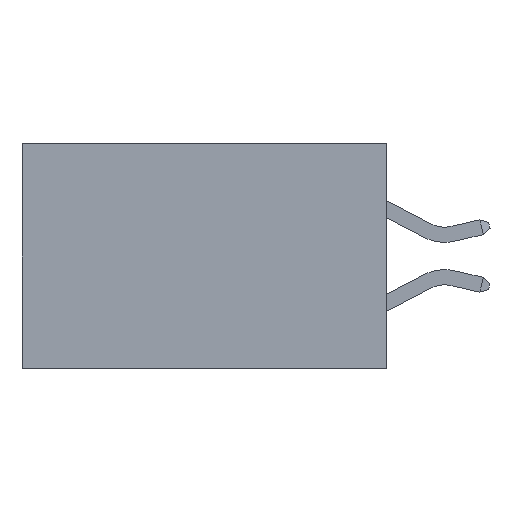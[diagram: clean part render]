
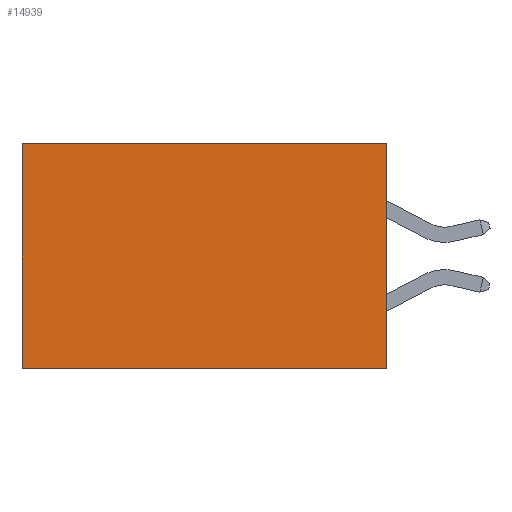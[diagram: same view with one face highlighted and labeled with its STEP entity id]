
A CAD part, left-side view. The second image highlights one B-rep face of the part: STEP entity #14939.
In plain terms, the highlighted planar face has unit normal (-1, 0, 0).
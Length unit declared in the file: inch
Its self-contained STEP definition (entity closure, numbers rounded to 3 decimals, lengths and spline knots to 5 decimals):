
#363 = DIRECTION ( 'NONE',  ( 0., 0., -1. ) ) ;
#607 = PLANE ( 'NONE',  #3276 ) ;
#1369 = DIRECTION ( 'NONE',  ( 0., 0., -1. ) ) ;
#1417 = VECTOR ( 'NONE', #17277, 39.37008 ) ;
#1928 = ORIENTED_EDGE ( 'NONE', *, *, #10941, .F. ) ;
#2033 = VERTEX_POINT ( 'NONE', #20275 ) ;
#2263 = ORIENTED_EDGE ( 'NONE', *, *, #16621, .F. ) ;
#2738 = CARTESIAN_POINT ( 'NONE',  ( 0.2615, 0.6, -0.37 ) ) ;
#2892 = CARTESIAN_POINT ( 'NONE',  ( 0.2615, 0., 0. ) ) ;
#3276 = AXIS2_PLACEMENT_3D ( 'NONE', #5854, #5934, #17933 ) ;
#3591 = VECTOR ( 'NONE', #17488, 39.37008 ) ;
#3689 = CARTESIAN_POINT ( 'NONE',  ( 0.2615, 0., 0. ) ) ;
#5116 = ORIENTED_EDGE ( 'NONE', *, *, #8542, .T. ) ;
#5854 = CARTESIAN_POINT ( 'NONE',  ( 0.2615, 0., -0.37 ) ) ;
#5934 = DIRECTION ( 'NONE',  ( 1., 0., 0. ) ) ;
#6112 = LINE ( 'NONE', #15629, #1417 ) ;
#6464 = EDGE_CURVE ( 'NONE', #15742, #2033, #12891, .T. ) ;
#7139 = FACE_OUTER_BOUND ( 'NONE', #9864, .T. ) ;
#7399 = LINE ( 'NONE', #10136, #21016 ) ;
#8137 = LINE ( 'NONE', #12625, #17184 ) ;
#8542 = EDGE_CURVE ( 'NONE', #2033, #15707, #7399, .T. ) ;
#9864 = EDGE_LOOP ( 'NONE', ( #5116, #2263, #1928, #19498 ) ) ;
#10136 = CARTESIAN_POINT ( 'NONE',  ( 0.2615, 0.6, -0.37 ) ) ;
#10637 = VERTEX_POINT ( 'NONE', #18699 ) ;
#10941 = EDGE_CURVE ( 'NONE', #15742, #10637, #8137, .T. ) ;
#12625 = CARTESIAN_POINT ( 'NONE',  ( 0.2615, 0., -0.37 ) ) ;
#12891 = LINE ( 'NONE', #3689, #3591 ) ;
#14939 = ADVANCED_FACE ( 'NONE', ( #7139 ), #607, .F. ) ;
#15629 = CARTESIAN_POINT ( 'NONE',  ( 0.2615, 0., -0.37 ) ) ;
#15707 = VERTEX_POINT ( 'NONE', #2738 ) ;
#15742 = VERTEX_POINT ( 'NONE', #2892 ) ;
#16621 = EDGE_CURVE ( 'NONE', #10637, #15707, #6112, .T. ) ;
#17184 = VECTOR ( 'NONE', #363, 39.37008 ) ;
#17277 = DIRECTION ( 'NONE',  ( 0., 1., 0. ) ) ;
#17488 = DIRECTION ( 'NONE',  ( 0., 1., 0. ) ) ;
#17933 = DIRECTION ( 'NONE',  ( 0., 0., -1. ) ) ;
#18699 = CARTESIAN_POINT ( 'NONE',  ( 0.2615, 0., -0.37 ) ) ;
#19498 = ORIENTED_EDGE ( 'NONE', *, *, #6464, .T. ) ;
#20275 = CARTESIAN_POINT ( 'NONE',  ( 0.2615, 0.6, 0. ) ) ;
#21016 = VECTOR ( 'NONE', #1369, 39.37008 ) ;
